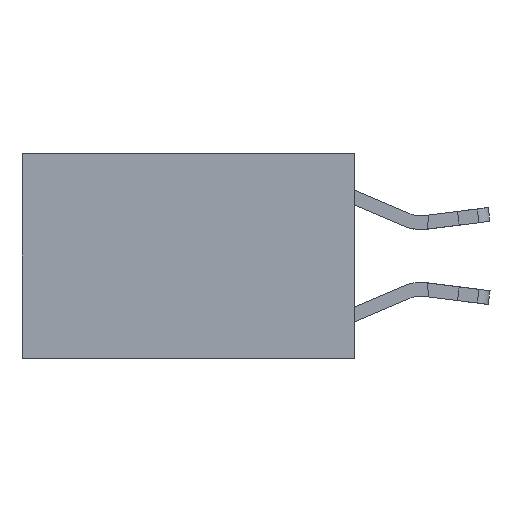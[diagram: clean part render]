
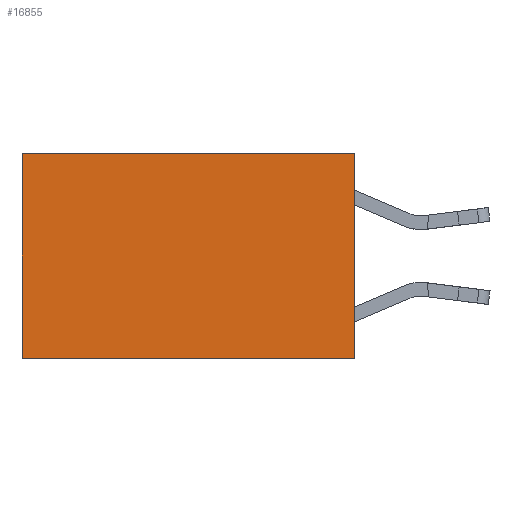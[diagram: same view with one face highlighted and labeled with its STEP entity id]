
A CAD part, left-side view. The second image highlights one B-rep face of the part: STEP entity #16855.
In plain terms, the highlighted planar face has unit normal (-1, 0, 0).
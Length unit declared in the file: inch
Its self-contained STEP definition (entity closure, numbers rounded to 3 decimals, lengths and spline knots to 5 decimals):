
#214 = EDGE_CURVE ( 'NONE', #18462, #15237, #505, .T. ) ;
#505 = LINE ( 'NONE', #17132, #18032 ) ;
#572 = VECTOR ( 'NONE', #19580, 39.37008 ) ;
#646 = CARTESIAN_POINT ( 'NONE',  ( 0.2625, 0., 0. ) ) ;
#1912 = LINE ( 'NONE', #646, #20223 ) ;
#3280 = CARTESIAN_POINT ( 'NONE',  ( 0.2625, 0., 0. ) ) ;
#4197 = CARTESIAN_POINT ( 'NONE',  ( 0.2625, 0.6, 0. ) ) ;
#5374 = CARTESIAN_POINT ( 'NONE',  ( 0.2625, 0.6, 0. ) ) ;
#5623 = EDGE_LOOP ( 'NONE', ( #17403, #11227, #11925, #23105 ) ) ;
#7256 = DIRECTION ( 'NONE',  ( 0., 0., -1. ) ) ;
#7587 = CARTESIAN_POINT ( 'NONE',  ( 0.2625, 0., 0. ) ) ;
#8786 = CARTESIAN_POINT ( 'NONE',  ( 0.2625, 0., -0.37 ) ) ;
#9468 = DIRECTION ( 'NONE',  ( 0., 0., -1. ) ) ;
#10450 = LINE ( 'NONE', #3280, #572 ) ;
#11219 = DIRECTION ( 'NONE',  ( 1., 0., 0. ) ) ;
#11227 = ORIENTED_EDGE ( 'NONE', *, *, #214, .F. ) ;
#11925 = ORIENTED_EDGE ( 'NONE', *, *, #11970, .F. ) ;
#11970 = EDGE_CURVE ( 'NONE', #20606, #18462, #1912, .T. ) ;
#12616 = CARTESIAN_POINT ( 'NONE',  ( 0.2625, 0., 0. ) ) ;
#12962 = PLANE ( 'NONE',  #14127 ) ;
#14127 = AXIS2_PLACEMENT_3D ( 'NONE', #7587, #11219, #9468 ) ;
#15237 = VERTEX_POINT ( 'NONE', #22774 ) ;
#15399 = DIRECTION ( 'NONE',  ( 0., 0., -1. ) ) ;
#15811 = DIRECTION ( 'NONE',  ( 0., 1., 0. ) ) ;
#15989 = EDGE_CURVE ( 'NONE', #20606, #16818, #10450, .T. ) ;
#16818 = VERTEX_POINT ( 'NONE', #4197 ) ;
#16855 = ADVANCED_FACE ( 'NONE', ( #20607 ), #12962, .F. ) ;
#17132 = CARTESIAN_POINT ( 'NONE',  ( 0.2625, 0., -0.37 ) ) ;
#17403 = ORIENTED_EDGE ( 'NONE', *, *, #19283, .T. ) ;
#17686 = VECTOR ( 'NONE', #7256, 39.37008 ) ;
#18032 = VECTOR ( 'NONE', #15811, 39.37008 ) ;
#18462 = VERTEX_POINT ( 'NONE', #8786 ) ;
#19283 = EDGE_CURVE ( 'NONE', #16818, #15237, #21906, .T. ) ;
#19580 = DIRECTION ( 'NONE',  ( 0., 1., 0. ) ) ;
#20223 = VECTOR ( 'NONE', #15399, 39.37008 ) ;
#20606 = VERTEX_POINT ( 'NONE', #12616 ) ;
#20607 = FACE_OUTER_BOUND ( 'NONE', #5623, .T. ) ;
#21906 = LINE ( 'NONE', #5374, #17686 ) ;
#22774 = CARTESIAN_POINT ( 'NONE',  ( 0.2625, 0.6, -0.37 ) ) ;
#23105 = ORIENTED_EDGE ( 'NONE', *, *, #15989, .T. ) ;
